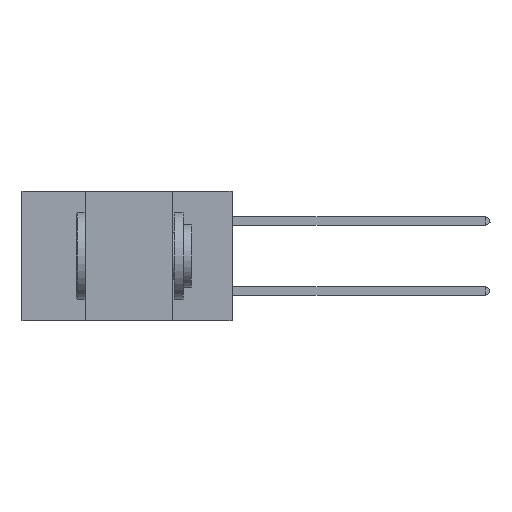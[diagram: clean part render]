
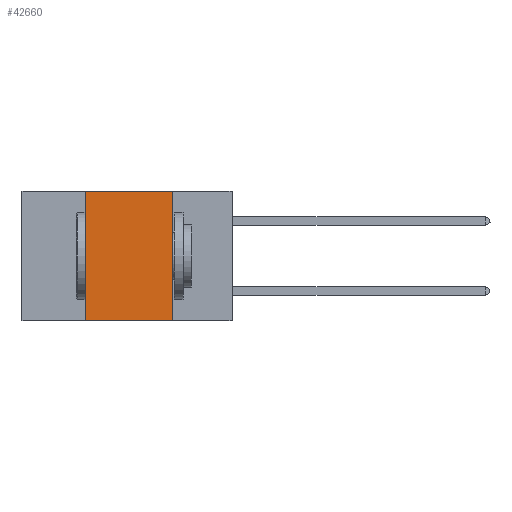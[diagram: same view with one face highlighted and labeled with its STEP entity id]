
A CAD part, left-side view. The second image highlights one B-rep face of the part: STEP entity #42660.
In plain terms, the highlighted planar face has unit normal (-1, 0, 0).
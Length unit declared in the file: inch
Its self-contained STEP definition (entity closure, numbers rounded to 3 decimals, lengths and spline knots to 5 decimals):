
#1118 = CARTESIAN_POINT ( 'NONE',  ( 0., 0.6, 0. ) ) ;
#3251 = ORIENTED_EDGE ( 'NONE', *, *, #31624, .F. ) ;
#3416 = CARTESIAN_POINT ( 'NONE',  ( 0., 0.17, -0.37 ) ) ;
#4070 = EDGE_LOOP ( 'NONE', ( #3251, #4145, #40129, #36449 ) ) ;
#4145 = ORIENTED_EDGE ( 'NONE', *, *, #30117, .F. ) ;
#4686 = VECTOR ( 'NONE', #42280, 39.37008 ) ;
#5837 = LINE ( 'NONE', #12352, #4686 ) ;
#7374 = VECTOR ( 'NONE', #36599, 39.37008 ) ;
#8129 = AXIS2_PLACEMENT_3D ( 'NONE', #1118, #41781, #19831 ) ;
#8802 = LINE ( 'NONE', #11149, #44902 ) ;
#11149 = CARTESIAN_POINT ( 'NONE',  ( 0., 0.6, -0.37 ) ) ;
#12352 = CARTESIAN_POINT ( 'NONE',  ( 0., 0.17, 0. ) ) ;
#12483 = PLANE ( 'NONE',  #8129 ) ;
#19831 = DIRECTION ( 'NONE',  ( 0., 0., -1. ) ) ;
#20233 = DIRECTION ( 'NONE',  ( 0., 0., 1. ) ) ;
#22229 = EDGE_CURVE ( 'NONE', #37867, #39450, #30421, .T. ) ;
#26869 = LINE ( 'NONE', #47379, #7374 ) ;
#28111 = VERTEX_POINT ( 'NONE', #3416 ) ;
#30117 = EDGE_CURVE ( 'NONE', #39450, #36078, #26869, .T. ) ;
#30421 = LINE ( 'NONE', #42819, #46420 ) ;
#31624 = EDGE_CURVE ( 'NONE', #36078, #28111, #5837, .T. ) ;
#36078 = VERTEX_POINT ( 'NONE', #42901 ) ;
#36449 = ORIENTED_EDGE ( 'NONE', *, *, #44969, .T. ) ;
#36599 = DIRECTION ( 'NONE',  ( 0., -1., 0. ) ) ;
#37867 = VERTEX_POINT ( 'NONE', #41493 ) ;
#39450 = VERTEX_POINT ( 'NONE', #42585 ) ;
#40129 = ORIENTED_EDGE ( 'NONE', *, *, #22229, .F. ) ;
#40725 = FACE_OUTER_BOUND ( 'NONE', #4070, .T. ) ;
#40768 = DIRECTION ( 'NONE',  ( 0., -1., 0. ) ) ;
#41493 = CARTESIAN_POINT ( 'NONE',  ( 0., 0.42, -0.37 ) ) ;
#41781 = DIRECTION ( 'NONE',  ( 1., 0., 0. ) ) ;
#42280 = DIRECTION ( 'NONE',  ( 0., 0., -1. ) ) ;
#42585 = CARTESIAN_POINT ( 'NONE',  ( 0., 0.42, 0. ) ) ;
#42660 = ADVANCED_FACE ( 'NONE', ( #40725 ), #12483, .F. ) ;
#42819 = CARTESIAN_POINT ( 'NONE',  ( 0., 0.42, 0. ) ) ;
#42901 = CARTESIAN_POINT ( 'NONE',  ( 0., 0.17, 0. ) ) ;
#44902 = VECTOR ( 'NONE', #40768, 39.37008 ) ;
#44969 = EDGE_CURVE ( 'NONE', #37867, #28111, #8802, .T. ) ;
#46420 = VECTOR ( 'NONE', #20233, 39.37008 ) ;
#47379 = CARTESIAN_POINT ( 'NONE',  ( 0., 0.6, 0. ) ) ;
